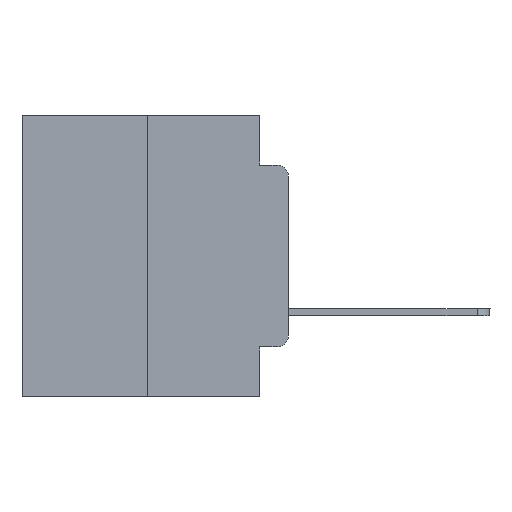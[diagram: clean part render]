
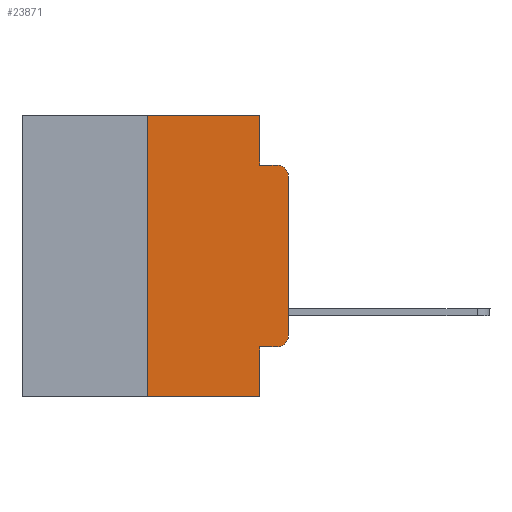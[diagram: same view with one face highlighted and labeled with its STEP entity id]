
A CAD part, left-side view. The second image highlights one B-rep face of the part: STEP entity #23871.
In plain terms, the highlighted planar face has unit normal (-1, 0, 0).
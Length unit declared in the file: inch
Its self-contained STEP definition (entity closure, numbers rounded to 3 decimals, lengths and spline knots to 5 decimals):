
#118 = CARTESIAN_POINT ( 'NONE',  ( 0., 0.051, 0. ) ) ;
#150 = ORIENTED_EDGE ( 'NONE', *, *, #17788, .T. ) ;
#428 = DIRECTION ( 'NONE',  ( 0., 0., -1. ) ) ;
#499 = FACE_OUTER_BOUND ( 'NONE', #3708, .T. ) ;
#667 = DIRECTION ( 'NONE',  ( 0., -1., 0. ) ) ;
#740 = LINE ( 'NONE', #1739, #6901 ) ;
#1739 = CARTESIAN_POINT ( 'NONE',  ( 0., 0.25, 0. ) ) ;
#1946 = ORIENTED_EDGE ( 'NONE', *, *, #11934, .T. ) ;
#2280 = VECTOR ( 'NONE', #24427, 39.37008 ) ;
#2443 = CARTESIAN_POINT ( 'NONE',  ( 0., 0., -0.1085 ) ) ;
#2664 = ORIENTED_EDGE ( 'NONE', *, *, #5539, .F. ) ;
#2682 = DIRECTION ( 'NONE',  ( 0., 0., 1. ) ) ;
#2821 = CARTESIAN_POINT ( 'NONE',  ( 0., 0.051, -0.4115 ) ) ;
#3608 = VERTEX_POINT ( 'NONE', #2443 ) ;
#3708 = EDGE_LOOP ( 'NONE', ( #16285, #23198, #2664, #19414, #6830, #7249, #14147, #6832, #150, #1946 ) ) ;
#5096 = EDGE_CURVE ( 'NONE', #6735, #21813, #21189, .T. ) ;
#5379 = CARTESIAN_POINT ( 'NONE',  ( 0., 0.02, -0.4115 ) ) ;
#5539 = EDGE_CURVE ( 'NONE', #24181, #10976, #10933, .T. ) ;
#6342 = VERTEX_POINT ( 'NONE', #17750 ) ;
#6735 = VERTEX_POINT ( 'NONE', #7617 ) ;
#6830 = ORIENTED_EDGE ( 'NONE', *, *, #14948, .F. ) ;
#6832 = ORIENTED_EDGE ( 'NONE', *, *, #5096, .F. ) ;
#6901 = VECTOR ( 'NONE', #25593, 39.37008 ) ;
#7249 = ORIENTED_EDGE ( 'NONE', *, *, #10904, .F. ) ;
#7267 = CARTESIAN_POINT ( 'NONE',  ( 0., 0.051, -0.0885 ) ) ;
#7328 = VERTEX_POINT ( 'NONE', #12713 ) ;
#7347 = VECTOR ( 'NONE', #8386, 39.37008 ) ;
#7617 = CARTESIAN_POINT ( 'NONE',  ( 0., 0.051, -0.4115 ) ) ;
#7671 = CARTESIAN_POINT ( 'NONE',  ( 0., 0.051, 0. ) ) ;
#8094 = CIRCLE ( 'NONE', #25359, 0.02 ) ;
#8150 = CARTESIAN_POINT ( 'NONE',  ( 0., 0., 0. ) ) ;
#8189 = VERTEX_POINT ( 'NONE', #25578 ) ;
#8386 = DIRECTION ( 'NONE',  ( 0., -1., 0. ) ) ;
#9986 = DIRECTION ( 'NONE',  ( 1., 0., 0. ) ) ;
#10171 = DIRECTION ( 'NONE',  ( 0., 0., -1. ) ) ;
#10517 = CIRCLE ( 'NONE', #18853, 0.02 ) ;
#10904 = EDGE_CURVE ( 'NONE', #11882, #6342, #740, .T. ) ;
#10933 = LINE ( 'NONE', #7267, #17452 ) ;
#10970 = DIRECTION ( 'NONE',  ( -1., 0., 0. ) ) ;
#10976 = VERTEX_POINT ( 'NONE', #22061 ) ;
#11352 = LINE ( 'NONE', #2821, #20651 ) ;
#11468 = DIRECTION ( 'NONE',  ( 0., -1., 0. ) ) ;
#11882 = VERTEX_POINT ( 'NONE', #24488 ) ;
#11934 = EDGE_CURVE ( 'NONE', #25547, #7328, #10517, .T. ) ;
#12713 = CARTESIAN_POINT ( 'NONE',  ( 0., 0., -0.3915 ) ) ;
#13751 = VECTOR ( 'NONE', #20077, 39.37008 ) ;
#14117 = EDGE_CURVE ( 'NONE', #7328, #3608, #16283, .T. ) ;
#14147 = ORIENTED_EDGE ( 'NONE', *, *, #22440, .T. ) ;
#14566 = CARTESIAN_POINT ( 'NONE',  ( 0., 0.473, -0.5 ) ) ;
#14779 = CARTESIAN_POINT ( 'NONE',  ( 0., 0.02, -0.3915 ) ) ;
#14938 = DIRECTION ( 'NONE',  ( 0., 0., -1. ) ) ;
#14948 = EDGE_CURVE ( 'NONE', #6342, #8189, #21833, .T. ) ;
#16092 = EDGE_CURVE ( 'NONE', #3608, #10976, #8094, .T. ) ;
#16283 = LINE ( 'NONE', #8150, #22174 ) ;
#16285 = ORIENTED_EDGE ( 'NONE', *, *, #14117, .T. ) ;
#16533 = CARTESIAN_POINT ( 'NONE',  ( 0., 0.473, 0. ) ) ;
#17452 = VECTOR ( 'NONE', #11468, 39.37008 ) ;
#17750 = CARTESIAN_POINT ( 'NONE',  ( 0., 0.25, 0. ) ) ;
#17788 = EDGE_CURVE ( 'NONE', #6735, #25547, #11352, .T. ) ;
#18574 = LINE ( 'NONE', #7671, #19813 ) ;
#18853 = AXIS2_PLACEMENT_3D ( 'NONE', #14779, #10970, #14938 ) ;
#19414 = ORIENTED_EDGE ( 'NONE', *, *, #22736, .F. ) ;
#19813 = VECTOR ( 'NONE', #23823, 39.37008 ) ;
#20077 = DIRECTION ( 'NONE',  ( 0., 0., -1. ) ) ;
#20234 = CARTESIAN_POINT ( 'NONE',  ( 0., 0.02, -0.1085 ) ) ;
#20651 = VECTOR ( 'NONE', #667, 39.37008 ) ;
#20652 = CARTESIAN_POINT ( 'NONE',  ( 0., 0.051, -0.0885 ) ) ;
#20844 = CARTESIAN_POINT ( 'NONE',  ( 0., 0.051, -0.5 ) ) ;
#21189 = LINE ( 'NONE', #118, #13751 ) ;
#21519 = PLANE ( 'NONE',  #23857 ) ;
#21813 = VERTEX_POINT ( 'NONE', #20844 ) ;
#21833 = LINE ( 'NONE', #16533, #2280 ) ;
#21878 = CARTESIAN_POINT ( 'NONE',  ( 0., 0.473, 0. ) ) ;
#22061 = CARTESIAN_POINT ( 'NONE',  ( 0., 0.02, -0.0885 ) ) ;
#22174 = VECTOR ( 'NONE', #2682, 39.37008 ) ;
#22440 = EDGE_CURVE ( 'NONE', #11882, #21813, #23834, .T. ) ;
#22736 = EDGE_CURVE ( 'NONE', #8189, #24181, #18574, .T. ) ;
#23198 = ORIENTED_EDGE ( 'NONE', *, *, #16092, .T. ) ;
#23823 = DIRECTION ( 'NONE',  ( 0., 0., -1. ) ) ;
#23834 = LINE ( 'NONE', #14566, #7347 ) ;
#23857 = AXIS2_PLACEMENT_3D ( 'NONE', #21878, #9986, #10171 ) ;
#23871 = ADVANCED_FACE ( 'NONE', ( #499 ), #21519, .F. ) ;
#24181 = VERTEX_POINT ( 'NONE', #20652 ) ;
#24206 = DIRECTION ( 'NONE',  ( -1., 0., 0. ) ) ;
#24427 = DIRECTION ( 'NONE',  ( 0., -1., 0. ) ) ;
#24488 = CARTESIAN_POINT ( 'NONE',  ( 0., 0.25, -0.5 ) ) ;
#25359 = AXIS2_PLACEMENT_3D ( 'NONE', #20234, #24206, #428 ) ;
#25547 = VERTEX_POINT ( 'NONE', #5379 ) ;
#25578 = CARTESIAN_POINT ( 'NONE',  ( 0., 0.051, 0. ) ) ;
#25593 = DIRECTION ( 'NONE',  ( 0., 0., 1. ) ) ;
